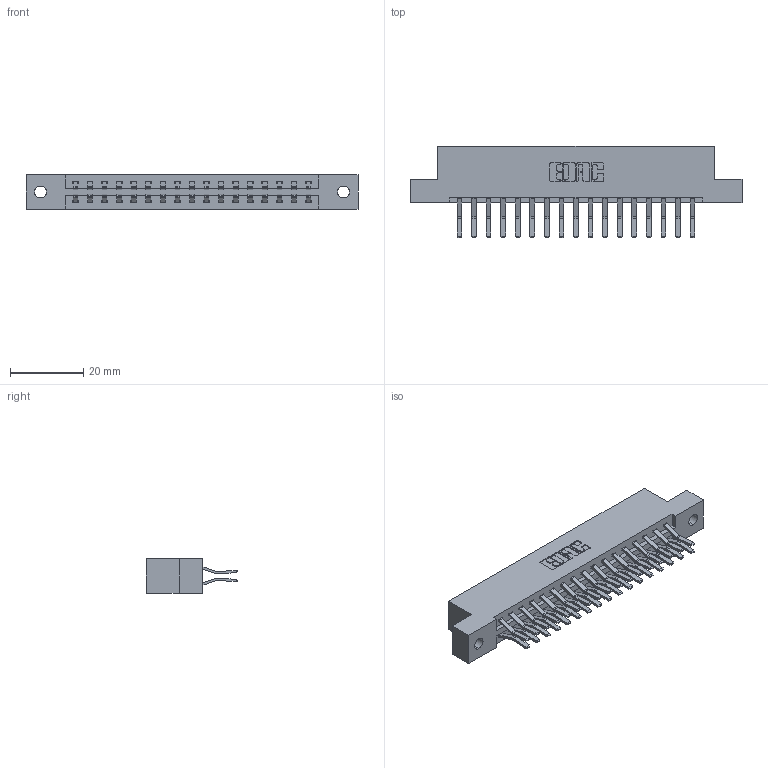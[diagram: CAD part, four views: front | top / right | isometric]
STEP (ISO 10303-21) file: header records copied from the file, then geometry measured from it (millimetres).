
FILE_DESCRIPTION (( 'STEP AP203' ), '1' );
FILE_NAME ('387-034-560-202.STEP', '2019-10-17T18:27:54', ( '' ), ( '' ), 'SwSTEP 2.0', 'SolidWorks 2016', '' );
FILE_SCHEMA (( 'CONFIG_CONTROL_DESIGN' ));
Length unit declared in the file: inch
Products named in the file (3): 345-292-001_560 Tail; 387-034-560-202; 337 Part_Flush Mounting Lugs - 0.128 Dia
Assembly tree (35 placements, depth 2):
  387-034-560-202
    337 Part_Flush Mounting Lugs - 0.128 Dia
    345-292-001_560 Tail  x34
Bounding box: 90.37 x 24.78 x 9.4 mm (x, y, z)
Volume: 9377.6 mm3; surface area: 10730.9 mm2
Topology: 35 solids, 35 shells, 2018 faces, 5989 edges, 3946 vertices
Faces by surface type: plane 1362, cylinder 656
Entity records: 16505 total; most frequent: CARTESIAN_POINT 2802, ORIENTED_EDGE 2738, DIRECTION 2433, EDGE_CURVE 1369, VECTOR 1237, LINE 1237, VERTEX_POINT 910, AXIS2_PLACEMENT_3D 598
